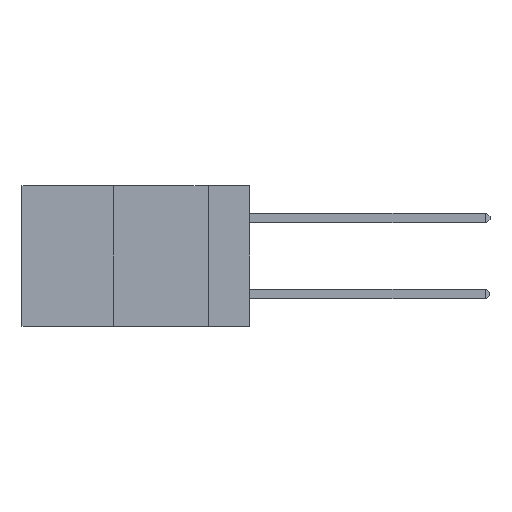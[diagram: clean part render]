
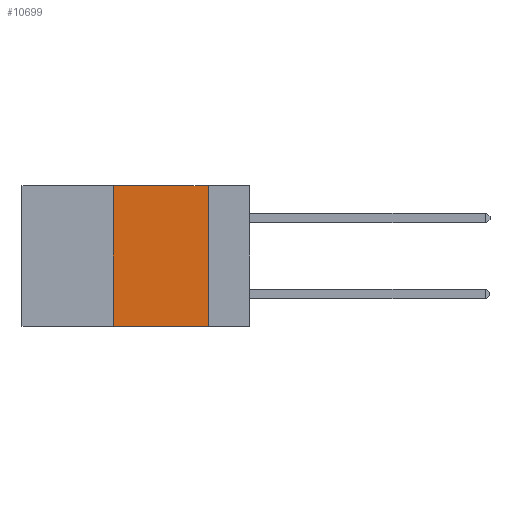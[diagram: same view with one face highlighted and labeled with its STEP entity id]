
A CAD part, left-side view. The second image highlights one B-rep face of the part: STEP entity #10699.
In plain terms, the highlighted planar face has unit normal (-1, 0, 0).
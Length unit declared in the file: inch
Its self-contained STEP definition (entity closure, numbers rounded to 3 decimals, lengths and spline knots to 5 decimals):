
#289 = ORIENTED_EDGE ( 'NONE', *, *, #1078, .F. ) ;
#345 = ORIENTED_EDGE ( 'NONE', *, *, #6919, .F. ) ;
#379 = ORIENTED_EDGE ( 'NONE', *, *, #6101, .F. ) ;
#445 = ORIENTED_EDGE ( 'NONE', *, *, #10549, .T. ) ;
#640 = CARTESIAN_POINT ( 'NONE',  ( 0., 0.36, 0. ) ) ;
#763 = VECTOR ( 'NONE', #4442, 39.37008 ) ;
#1049 = DIRECTION ( 'NONE',  ( 0., -1., 0. ) ) ;
#1078 = EDGE_CURVE ( 'NONE', #7482, #10633, #5449, .T. ) ;
#1257 = VERTEX_POINT ( 'NONE', #1389 ) ;
#1389 = CARTESIAN_POINT ( 'NONE',  ( 0., 0.36, -0.37 ) ) ;
#1704 = EDGE_LOOP ( 'NONE', ( #289, #345, #379, #445 ) ) ;
#1857 = VECTOR ( 'NONE', #1049, 39.37008 ) ;
#2153 = LINE ( 'NONE', #7926, #1857 ) ;
#2238 = PLANE ( 'NONE',  #4497 ) ;
#2243 = FACE_OUTER_BOUND ( 'NONE', #1704, .T. ) ;
#3058 = LINE ( 'NONE', #8756, #9203 ) ;
#3076 = DIRECTION ( 'NONE',  ( 0., 0., -1. ) ) ;
#3400 = DIRECTION ( 'NONE',  ( 0., 0., 1. ) ) ;
#4442 = DIRECTION ( 'NONE',  ( 0., 0., -1. ) ) ;
#4497 = AXIS2_PLACEMENT_3D ( 'NONE', #5598, #8128, #3076 ) ;
#4526 = CARTESIAN_POINT ( 'NONE',  ( 0., 0.11, 0. ) ) ;
#4812 = LINE ( 'NONE', #640, #8721 ) ;
#5449 = LINE ( 'NONE', #4526, #763 ) ;
#5598 = CARTESIAN_POINT ( 'NONE',  ( 0., 0.6, 0. ) ) ;
#6101 = EDGE_CURVE ( 'NONE', #1257, #6986, #4812, .T. ) ;
#6385 = CARTESIAN_POINT ( 'NONE',  ( 0., 0.36, 0. ) ) ;
#6919 = EDGE_CURVE ( 'NONE', #6986, #7482, #3058, .T. ) ;
#6986 = VERTEX_POINT ( 'NONE', #6385 ) ;
#7139 = CARTESIAN_POINT ( 'NONE',  ( 0., 0.11, -0.37 ) ) ;
#7482 = VERTEX_POINT ( 'NONE', #9306 ) ;
#7926 = CARTESIAN_POINT ( 'NONE',  ( 0., 0.6, -0.37 ) ) ;
#8128 = DIRECTION ( 'NONE',  ( 1., 0., 0. ) ) ;
#8721 = VECTOR ( 'NONE', #3400, 39.37008 ) ;
#8756 = CARTESIAN_POINT ( 'NONE',  ( 0., 0.6, 0. ) ) ;
#9203 = VECTOR ( 'NONE', #9554, 39.37008 ) ;
#9306 = CARTESIAN_POINT ( 'NONE',  ( 0., 0.11, 0. ) ) ;
#9554 = DIRECTION ( 'NONE',  ( 0., -1., 0. ) ) ;
#10549 = EDGE_CURVE ( 'NONE', #1257, #10633, #2153, .T. ) ;
#10633 = VERTEX_POINT ( 'NONE', #7139 ) ;
#10699 = ADVANCED_FACE ( 'NONE', ( #2243 ), #2238, .F. ) ;
